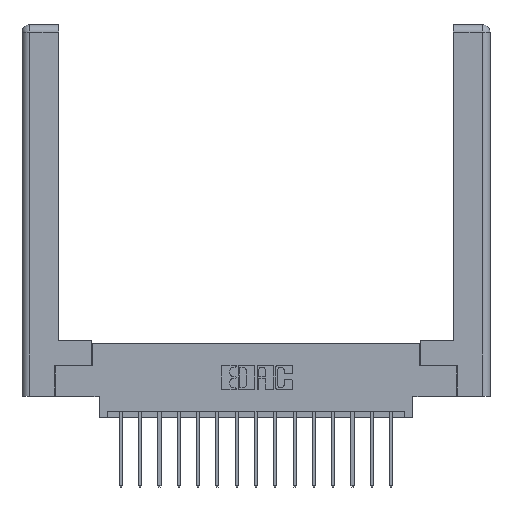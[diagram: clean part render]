
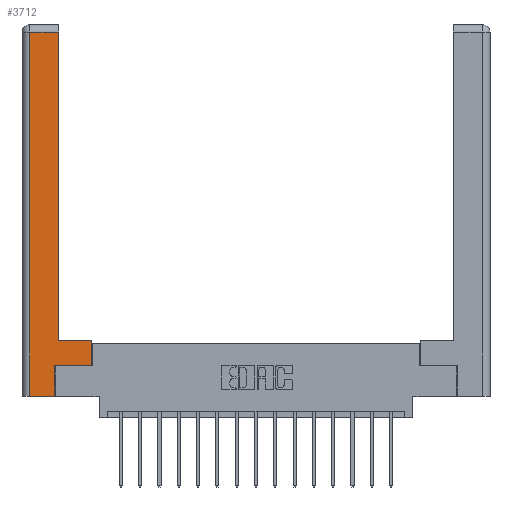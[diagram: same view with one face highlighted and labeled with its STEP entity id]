
A CAD part, top view. The second image highlights one B-rep face of the part: STEP entity #3712.
In plain terms, the highlighted planar face has unit normal (0, 0, 1).
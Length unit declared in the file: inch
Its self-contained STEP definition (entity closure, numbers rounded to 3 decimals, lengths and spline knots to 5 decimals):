
#624 = CARTESIAN_POINT ( 'NONE',  ( 0.565, 0.245, 0. ) ) ;
#916 = EDGE_CURVE ( 'NONE', #2061, #1043, #16361, .T. ) ;
#1043 = VERTEX_POINT ( 'NONE', #7226 ) ;
#1122 = VECTOR ( 'NONE', #4615, 39.37008 ) ;
#1211 = LINE ( 'NONE', #13157, #16802 ) ;
#1587 = VERTEX_POINT ( 'NONE', #9664 ) ;
#1848 = VERTEX_POINT ( 'NONE', #17579 ) ;
#2061 = VERTEX_POINT ( 'NONE', #8198 ) ;
#2185 = ORIENTED_EDGE ( 'NONE', *, *, #12483, .T. ) ;
#2271 = VECTOR ( 'NONE', #11207, 39.37008 ) ;
#2528 = DIRECTION ( 'NONE',  ( 0., 1., 0. ) ) ;
#2661 = VECTOR ( 'NONE', #2528, 39.37008 ) ;
#2670 = EDGE_CURVE ( 'NONE', #1848, #9720, #7628, .T. ) ;
#2735 = DIRECTION ( 'NONE',  ( -1., 0., 0. ) ) ;
#3331 = CARTESIAN_POINT ( 'NONE',  ( 0.295, 0.45, 0. ) ) ;
#3470 = CARTESIAN_POINT ( 'NONE',  ( 0.295, 0.45, 0. ) ) ;
#3494 = EDGE_LOOP ( 'NONE', ( #13654, #4006, #16833, #2185, #5581, #13553, #4485, #14776 ) ) ;
#3712 = ADVANCED_FACE ( 'NONE', ( #11714 ), #11046, .F. ) ;
#3771 = VERTEX_POINT ( 'NONE', #10804 ) ;
#4006 = ORIENTED_EDGE ( 'NONE', *, *, #5218, .T. ) ;
#4294 = LINE ( 'NONE', #11409, #6493 ) ;
#4485 = ORIENTED_EDGE ( 'NONE', *, *, #8311, .T. ) ;
#4513 = CARTESIAN_POINT ( 'NONE',  ( 0.265, 0.245, 0. ) ) ;
#4615 = DIRECTION ( 'NONE',  ( -1., 0., 0. ) ) ;
#5218 = EDGE_CURVE ( 'NONE', #3771, #2061, #4294, .T. ) ;
#5407 = CARTESIAN_POINT ( 'NONE',  ( 0., 0., 0. ) ) ;
#5581 = ORIENTED_EDGE ( 'NONE', *, *, #6889, .T. ) ;
#5923 = VECTOR ( 'NONE', #16324, 39.37008 ) ;
#6130 = LINE ( 'NONE', #17854, #2661 ) ;
#6493 = VECTOR ( 'NONE', #8883, 39.37008 ) ;
#6889 = EDGE_CURVE ( 'NONE', #1587, #10854, #12097, .T. ) ;
#7226 = CARTESIAN_POINT ( 'NONE',  ( 0.0615, 0., 0. ) ) ;
#7245 = DIRECTION ( 'NONE',  ( 1., 0., 0. ) ) ;
#7628 = LINE ( 'NONE', #3470, #1122 ) ;
#8010 = EDGE_CURVE ( 'NONE', #10854, #10444, #8768, .T. ) ;
#8094 = CARTESIAN_POINT ( 'NONE',  ( 0.265, 0.245, 0. ) ) ;
#8198 = CARTESIAN_POINT ( 'NONE',  ( 0.0615, 2.94, 0. ) ) ;
#8311 = EDGE_CURVE ( 'NONE', #10444, #1848, #6130, .T. ) ;
#8527 = VECTOR ( 'NONE', #7245, 39.37008 ) ;
#8768 = LINE ( 'NONE', #15593, #8527 ) ;
#8883 = DIRECTION ( 'NONE',  ( -1., 0., 0. ) ) ;
#8896 = AXIS2_PLACEMENT_3D ( 'NONE', #5407, #9653, #2735 ) ;
#9608 = LINE ( 'NONE', #16493, #5923 ) ;
#9653 = DIRECTION ( 'NONE',  ( 0., 0., -1. ) ) ;
#9664 = CARTESIAN_POINT ( 'NONE',  ( 0.265, 0., 0. ) ) ;
#9720 = VERTEX_POINT ( 'NONE', #3331 ) ;
#10121 = DIRECTION ( 'NONE',  ( 0., 1., 0. ) ) ;
#10444 = VERTEX_POINT ( 'NONE', #624 ) ;
#10804 = CARTESIAN_POINT ( 'NONE',  ( 0.295, 2.94, 0. ) ) ;
#10854 = VERTEX_POINT ( 'NONE', #4513 ) ;
#11046 = PLANE ( 'NONE',  #8896 ) ;
#11186 = EDGE_CURVE ( 'NONE', #9720, #3771, #1211, .T. ) ;
#11207 = DIRECTION ( 'NONE',  ( 0., -1., 0. ) ) ;
#11409 = CARTESIAN_POINT ( 'NONE',  ( 0.0615, 2.94, 0. ) ) ;
#11714 = FACE_OUTER_BOUND ( 'NONE', #3494, .T. ) ;
#12097 = LINE ( 'NONE', #8094, #14894 ) ;
#12483 = EDGE_CURVE ( 'NONE', #1043, #1587, #9608, .T. ) ;
#13157 = CARTESIAN_POINT ( 'NONE',  ( 0.295, 3., 0. ) ) ;
#13553 = ORIENTED_EDGE ( 'NONE', *, *, #8010, .T. ) ;
#13654 = ORIENTED_EDGE ( 'NONE', *, *, #11186, .T. ) ;
#14776 = ORIENTED_EDGE ( 'NONE', *, *, #2670, .T. ) ;
#14894 = VECTOR ( 'NONE', #16207, 39.37008 ) ;
#15593 = CARTESIAN_POINT ( 'NONE',  ( 0.565, 0.245, 0. ) ) ;
#16207 = DIRECTION ( 'NONE',  ( 0., 1., 0. ) ) ;
#16324 = DIRECTION ( 'NONE',  ( 1., 0., 0. ) ) ;
#16361 = LINE ( 'NONE', #16483, #2271 ) ;
#16483 = CARTESIAN_POINT ( 'NONE',  ( 0.0615, 0., 0. ) ) ;
#16493 = CARTESIAN_POINT ( 'NONE',  ( 0.265, 0., 0. ) ) ;
#16802 = VECTOR ( 'NONE', #10121, 39.37008 ) ;
#16833 = ORIENTED_EDGE ( 'NONE', *, *, #916, .T. ) ;
#17579 = CARTESIAN_POINT ( 'NONE',  ( 0.565, 0.45, 0. ) ) ;
#17854 = CARTESIAN_POINT ( 'NONE',  ( 0.565, 0.45, 0. ) ) ;
